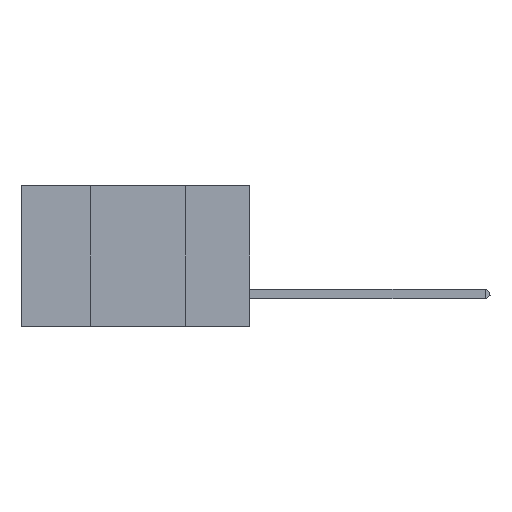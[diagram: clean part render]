
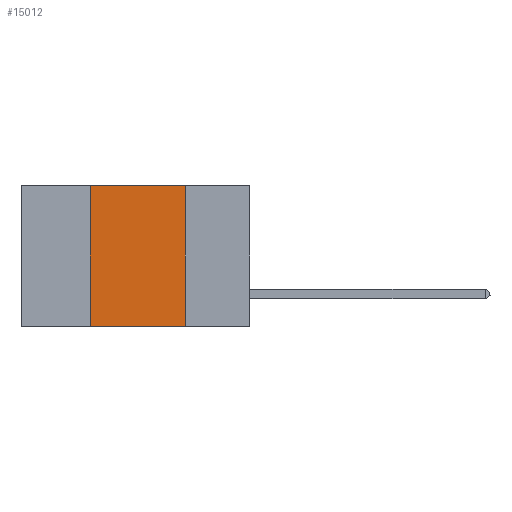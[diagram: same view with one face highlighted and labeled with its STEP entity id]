
A CAD part, left-side view. The second image highlights one B-rep face of the part: STEP entity #15012.
In plain terms, the highlighted planar face has unit normal (-1, 0, 0).
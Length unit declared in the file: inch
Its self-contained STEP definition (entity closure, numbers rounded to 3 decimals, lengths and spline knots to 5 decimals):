
#290 = VECTOR ( 'NONE', #10186, 39.37008 ) ;
#353 = DIRECTION ( 'NONE',  ( 0., -1., 0. ) ) ;
#1035 = CARTESIAN_POINT ( 'NONE',  ( 0., 0.17, -0.37 ) ) ;
#1370 = LINE ( 'NONE', #10784, #5931 ) ;
#1522 = DIRECTION ( 'NONE',  ( 0., 0., 1. ) ) ;
#1848 = EDGE_CURVE ( 'NONE', #12171, #15594, #8478, .T. ) ;
#3758 = ORIENTED_EDGE ( 'NONE', *, *, #1848, .F. ) ;
#4638 = EDGE_CURVE ( 'NONE', #11208, #12171, #1370, .T. ) ;
#5004 = ORIENTED_EDGE ( 'NONE', *, *, #4638, .F. ) ;
#5498 = CARTESIAN_POINT ( 'NONE',  ( 0., 0.6, 0. ) ) ;
#5931 = VECTOR ( 'NONE', #353, 39.37008 ) ;
#6075 = LINE ( 'NONE', #10792, #12589 ) ;
#6820 = VECTOR ( 'NONE', #9749, 39.37008 ) ;
#7083 = CARTESIAN_POINT ( 'NONE',  ( 0., 0.42, -0.37 ) ) ;
#7280 = EDGE_CURVE ( 'NONE', #19399, #15594, #16190, .T. ) ;
#7317 = EDGE_CURVE ( 'NONE', #19399, #11208, #6075, .T. ) ;
#7360 = FACE_OUTER_BOUND ( 'NONE', #7769, .T. ) ;
#7769 = EDGE_LOOP ( 'NONE', ( #3758, #5004, #8541, #14249 ) ) ;
#8478 = LINE ( 'NONE', #11810, #290 ) ;
#8541 = ORIENTED_EDGE ( 'NONE', *, *, #7317, .F. ) ;
#9749 = DIRECTION ( 'NONE',  ( 0., -1., 0. ) ) ;
#10186 = DIRECTION ( 'NONE',  ( 0., 0., -1. ) ) ;
#10784 = CARTESIAN_POINT ( 'NONE',  ( 0., 0.6, 0. ) ) ;
#10792 = CARTESIAN_POINT ( 'NONE',  ( 0., 0.42, 0. ) ) ;
#11208 = VERTEX_POINT ( 'NONE', #17979 ) ;
#11810 = CARTESIAN_POINT ( 'NONE',  ( 0., 0.17, 0. ) ) ;
#12171 = VERTEX_POINT ( 'NONE', #17813 ) ;
#12589 = VECTOR ( 'NONE', #1522, 39.37008 ) ;
#12980 = AXIS2_PLACEMENT_3D ( 'NONE', #5498, #17384, #19678 ) ;
#14249 = ORIENTED_EDGE ( 'NONE', *, *, #7280, .T. ) ;
#15012 = ADVANCED_FACE ( 'NONE', ( #7360 ), #17055, .F. ) ;
#15594 = VERTEX_POINT ( 'NONE', #1035 ) ;
#16190 = LINE ( 'NONE', #17641, #6820 ) ;
#17055 = PLANE ( 'NONE',  #12980 ) ;
#17384 = DIRECTION ( 'NONE',  ( 1., 0., 0. ) ) ;
#17641 = CARTESIAN_POINT ( 'NONE',  ( 0., 0.6, -0.37 ) ) ;
#17813 = CARTESIAN_POINT ( 'NONE',  ( 0., 0.17, 0. ) ) ;
#17979 = CARTESIAN_POINT ( 'NONE',  ( 0., 0.42, 0. ) ) ;
#19399 = VERTEX_POINT ( 'NONE', #7083 ) ;
#19678 = DIRECTION ( 'NONE',  ( 0., 0., -1. ) ) ;
